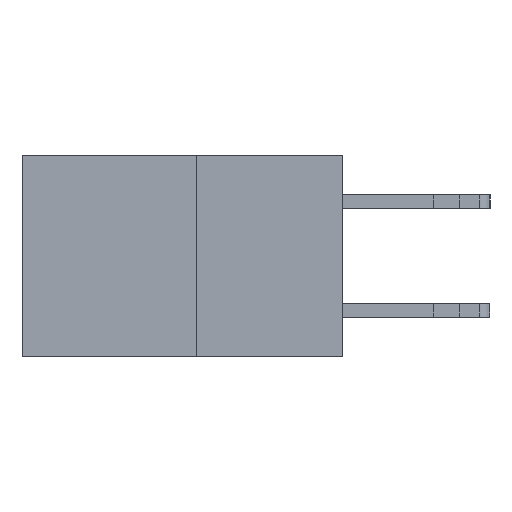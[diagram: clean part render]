
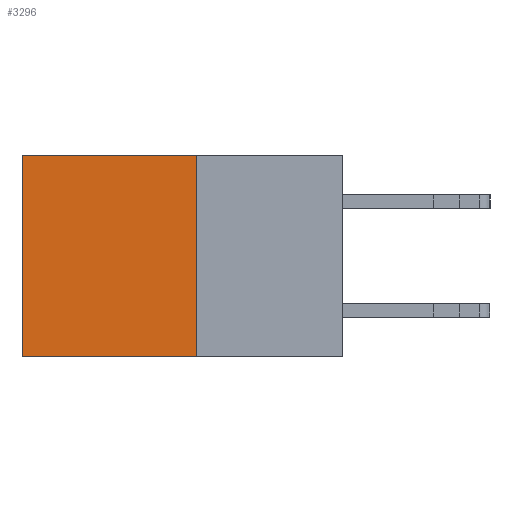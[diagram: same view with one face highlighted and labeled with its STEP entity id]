
A CAD part, left-side view. The second image highlights one B-rep face of the part: STEP entity #3296.
In plain terms, the highlighted planar face has unit normal (-1, 0, 0).
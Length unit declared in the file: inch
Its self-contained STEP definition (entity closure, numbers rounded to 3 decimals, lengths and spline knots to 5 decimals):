
#66 = AXIS2_PLACEMENT_3D ( 'NONE', #15397, #8139, #13091 ) ;
#975 = ORIENTED_EDGE ( 'NONE', *, *, #3320, .F. ) ;
#2306 = EDGE_CURVE ( 'NONE', #8247, #11232, #3332, .T. ) ;
#2425 = EDGE_LOOP ( 'NONE', ( #9074, #14188, #975, #14747 ) ) ;
#2686 = CARTESIAN_POINT ( 'NONE',  ( 0.277, 0.59, 0. ) ) ;
#3296 = ADVANCED_FACE ( 'NONE', ( #14914 ), #9678, .F. ) ;
#3320 = EDGE_CURVE ( 'NONE', #16835, #8247, #6270, .T. ) ;
#3331 = VERTEX_POINT ( 'NONE', #2686 ) ;
#3332 = LINE ( 'NONE', #13278, #7386 ) ;
#4272 = CARTESIAN_POINT ( 'NONE',  ( 0.277, 0.59, -0.37 ) ) ;
#5444 = EDGE_CURVE ( 'NONE', #3331, #11232, #16965, .T. ) ;
#6270 = LINE ( 'NONE', #20464, #18938 ) ;
#7386 = VECTOR ( 'NONE', #13025, 39.37008 ) ;
#8139 = DIRECTION ( 'NONE',  ( 1., 0., 0. ) ) ;
#8247 = VERTEX_POINT ( 'NONE', #8884 ) ;
#8884 = CARTESIAN_POINT ( 'NONE',  ( 0.277, 0.27, -0.37 ) ) ;
#9074 = ORIENTED_EDGE ( 'NONE', *, *, #5444, .T. ) ;
#9678 = PLANE ( 'NONE',  #66 ) ;
#10463 = DIRECTION ( 'NONE',  ( 0., 0., -1. ) ) ;
#11232 = VERTEX_POINT ( 'NONE', #4272 ) ;
#12348 = VECTOR ( 'NONE', #15557, 39.37008 ) ;
#13025 = DIRECTION ( 'NONE',  ( 0., 1., 0. ) ) ;
#13091 = DIRECTION ( 'NONE',  ( 0., 0., -1. ) ) ;
#13278 = CARTESIAN_POINT ( 'NONE',  ( 0.277, 0.27, -0.37 ) ) ;
#14188 = ORIENTED_EDGE ( 'NONE', *, *, #2306, .F. ) ;
#14747 = ORIENTED_EDGE ( 'NONE', *, *, #18035, .T. ) ;
#14914 = FACE_OUTER_BOUND ( 'NONE', #2425, .T. ) ;
#14989 = LINE ( 'NONE', #16837, #19004 ) ;
#15109 = DIRECTION ( 'NONE',  ( 0., 1., 0. ) ) ;
#15397 = CARTESIAN_POINT ( 'NONE',  ( 0.277, 0.27, -0.37 ) ) ;
#15557 = DIRECTION ( 'NONE',  ( 0., 0., -1. ) ) ;
#15693 = CARTESIAN_POINT ( 'NONE',  ( 0.277, 0.59, -0.37 ) ) ;
#16835 = VERTEX_POINT ( 'NONE', #18679 ) ;
#16837 = CARTESIAN_POINT ( 'NONE',  ( 0.277, 0.27, 0. ) ) ;
#16965 = LINE ( 'NONE', #15693, #12348 ) ;
#18035 = EDGE_CURVE ( 'NONE', #16835, #3331, #14989, .T. ) ;
#18679 = CARTESIAN_POINT ( 'NONE',  ( 0.277, 0.27, 0. ) ) ;
#18938 = VECTOR ( 'NONE', #10463, 39.37008 ) ;
#19004 = VECTOR ( 'NONE', #15109, 39.37008 ) ;
#20464 = CARTESIAN_POINT ( 'NONE',  ( 0.277, 0.27, -0.37 ) ) ;
